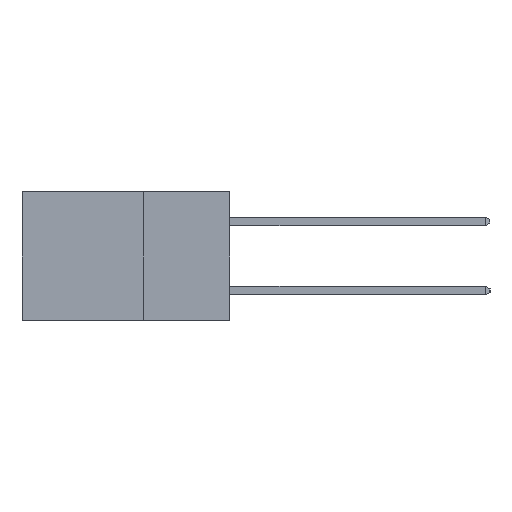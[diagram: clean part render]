
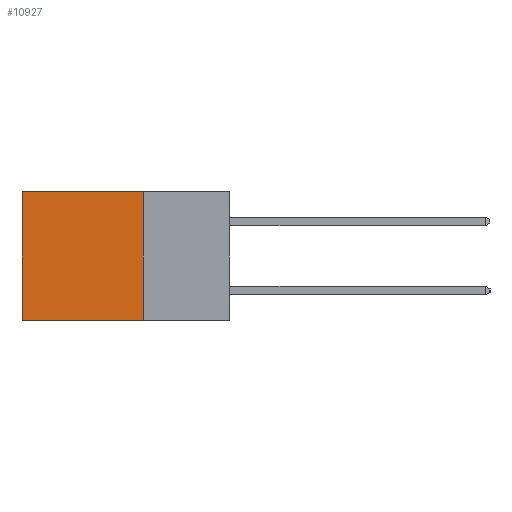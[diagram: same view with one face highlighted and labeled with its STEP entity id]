
A CAD part, left-side view. The second image highlights one B-rep face of the part: STEP entity #10927.
In plain terms, the highlighted planar face has unit normal (-1, 0, 0).
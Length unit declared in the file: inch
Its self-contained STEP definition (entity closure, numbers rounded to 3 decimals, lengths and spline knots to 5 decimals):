
#983 = ORIENTED_EDGE ( 'NONE', *, *, #9560, .F. ) ;
#1315 = DIRECTION ( 'NONE',  ( 0., 1., 0. ) ) ;
#2435 = EDGE_CURVE ( 'NONE', #12563, #18247, #14296, .T. ) ;
#3534 = DIRECTION ( 'NONE',  ( 1., 0., 0. ) ) ;
#3572 = ORIENTED_EDGE ( 'NONE', *, *, #16874, .F. ) ;
#3868 = EDGE_LOOP ( 'NONE', ( #14922, #3572, #983, #17300 ) ) ;
#5333 = DIRECTION ( 'NONE',  ( 0., 1., 0. ) ) ;
#6452 = DIRECTION ( 'NONE',  ( 0., 0., -1. ) ) ;
#7073 = FACE_OUTER_BOUND ( 'NONE', #3868, .T. ) ;
#8902 = CARTESIAN_POINT ( 'NONE',  ( 0.2615, 0.25, -0.37 ) ) ;
#9560 = EDGE_CURVE ( 'NONE', #12563, #15710, #20432, .T. ) ;
#10074 = CARTESIAN_POINT ( 'NONE',  ( 0.2615, 0.6, -0.37 ) ) ;
#10835 = CARTESIAN_POINT ( 'NONE',  ( 0.2615, 0.25, -0.37 ) ) ;
#10927 = ADVANCED_FACE ( 'NONE', ( #7073 ), #23470, .F. ) ;
#12019 = EDGE_CURVE ( 'NONE', #18247, #15072, #16935, .T. ) ;
#12438 = CARTESIAN_POINT ( 'NONE',  ( 0.2615, 0.25, -0.37 ) ) ;
#12530 = VECTOR ( 'NONE', #1315, 39.37008 ) ;
#12563 = VERTEX_POINT ( 'NONE', #19584 ) ;
#12569 = DIRECTION ( 'NONE',  ( 0., 0., -1. ) ) ;
#13875 = AXIS2_PLACEMENT_3D ( 'NONE', #10835, #3534, #16300 ) ;
#14296 = LINE ( 'NONE', #20577, #23313 ) ;
#14922 = ORIENTED_EDGE ( 'NONE', *, *, #12019, .T. ) ;
#15072 = VERTEX_POINT ( 'NONE', #19231 ) ;
#15643 = VECTOR ( 'NONE', #12569, 39.37008 ) ;
#15710 = VERTEX_POINT ( 'NONE', #20143 ) ;
#16249 = CARTESIAN_POINT ( 'NONE',  ( 0.2615, 0.6, 0. ) ) ;
#16300 = DIRECTION ( 'NONE',  ( 0., 0., -1. ) ) ;
#16353 = VECTOR ( 'NONE', #6452, 39.37008 ) ;
#16754 = LINE ( 'NONE', #12438, #12530 ) ;
#16874 = EDGE_CURVE ( 'NONE', #15710, #15072, #16754, .T. ) ;
#16935 = LINE ( 'NONE', #10074, #16353 ) ;
#17300 = ORIENTED_EDGE ( 'NONE', *, *, #2435, .T. ) ;
#18247 = VERTEX_POINT ( 'NONE', #16249 ) ;
#19231 = CARTESIAN_POINT ( 'NONE',  ( 0.2615, 0.6, -0.37 ) ) ;
#19584 = CARTESIAN_POINT ( 'NONE',  ( 0.2615, 0.25, 0. ) ) ;
#20143 = CARTESIAN_POINT ( 'NONE',  ( 0.2615, 0.25, -0.37 ) ) ;
#20432 = LINE ( 'NONE', #8902, #15643 ) ;
#20577 = CARTESIAN_POINT ( 'NONE',  ( 0.2615, 0.25, 0. ) ) ;
#23313 = VECTOR ( 'NONE', #5333, 39.37008 ) ;
#23470 = PLANE ( 'NONE',  #13875 ) ;
